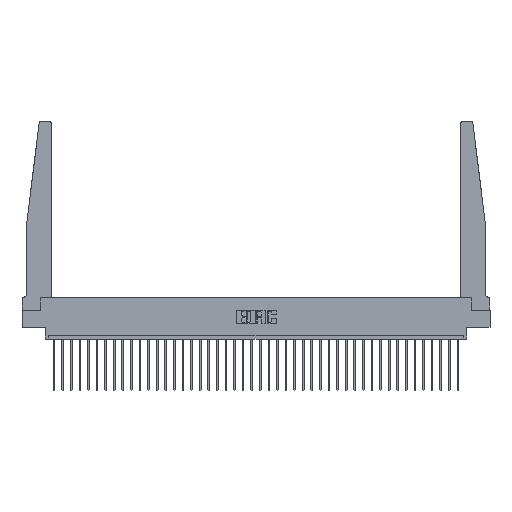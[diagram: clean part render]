
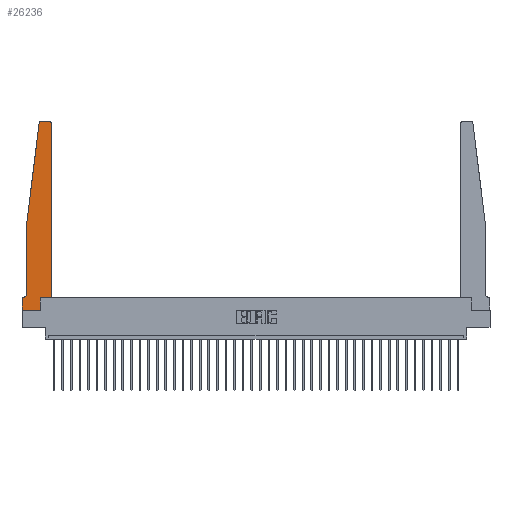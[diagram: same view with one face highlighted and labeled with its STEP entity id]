
A CAD part, top view. The second image highlights one B-rep face of the part: STEP entity #26236.
In plain terms, the highlighted planar face has unit normal (0, 0, 1).
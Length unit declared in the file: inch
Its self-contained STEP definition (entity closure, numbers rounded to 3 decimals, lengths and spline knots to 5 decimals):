
#259 = VECTOR ( 'NONE', #19504, 39.37008 ) ;
#717 = DIRECTION ( 'NONE',  ( 0., 0., 1. ) ) ;
#832 = ORIENTED_EDGE ( 'NONE', *, *, #10052, .T. ) ;
#1225 = VECTOR ( 'NONE', #22235, 39.37008 ) ;
#1252 = CARTESIAN_POINT ( 'NONE',  ( 0.015, 0.2375, 0.37 ) ) ;
#1656 = LINE ( 'NONE', #3688, #13061 ) ;
#1762 = EDGE_CURVE ( 'NONE', #8208, #15382, #31924, .T. ) ;
#2377 = CARTESIAN_POINT ( 'NONE',  ( 0., 0.1875, 0.37 ) ) ;
#2489 = LINE ( 'NONE', #8571, #6580 ) ;
#2525 = LINE ( 'NONE', #32675, #13989 ) ;
#3051 = ORIENTED_EDGE ( 'NONE', *, *, #27903, .T. ) ;
#3588 = ORIENTED_EDGE ( 'NONE', *, *, #18045, .T. ) ;
#3688 = CARTESIAN_POINT ( 'NONE',  ( 0., 0., 0.37 ) ) ;
#4366 = CARTESIAN_POINT ( 'NONE',  ( 0.425, 0.18, 0.37 ) ) ;
#4421 = CARTESIAN_POINT ( 'NONE',  ( 0.065, 0.1875, 0.37 ) ) ;
#4464 = VERTEX_POINT ( 'NONE', #14008 ) ;
#4659 = ORIENTED_EDGE ( 'NONE', *, *, #14331, .T. ) ;
#4847 = ORIENTED_EDGE ( 'NONE', *, *, #25561, .T. ) ;
#5660 = LINE ( 'NONE', #4421, #16729 ) ;
#5717 = VECTOR ( 'NONE', #11387, 39.37008 ) ;
#6159 = ORIENTED_EDGE ( 'NONE', *, *, #17369, .T. ) ;
#6405 = CARTESIAN_POINT ( 'NONE',  ( 0.065, 1.25, 0.37 ) ) ;
#6427 = VERTEX_POINT ( 'NONE', #22055 ) ;
#6580 = VECTOR ( 'NONE', #8460, 39.37008 ) ;
#7458 = DIRECTION ( 'NONE',  ( 0., 0., 1. ) ) ;
#7943 = VERTEX_POINT ( 'NONE', #2377 ) ;
#8208 = VERTEX_POINT ( 'NONE', #17450 ) ;
#8460 = DIRECTION ( 'NONE',  ( 0., -1., 0. ) ) ;
#8571 = CARTESIAN_POINT ( 'NONE',  ( 0.065, 1.25, 0.37 ) ) ;
#8684 = EDGE_CURVE ( 'NONE', #6427, #4464, #31117, .T. ) ;
#8844 = DIRECTION ( 'NONE',  ( 1., 0., 0. ) ) ;
#9470 = PLANE ( 'NONE',  #16461 ) ;
#9927 = CARTESIAN_POINT ( 'NONE',  ( 0.395, 2.75, 0.37 ) ) ;
#10019 = EDGE_CURVE ( 'NONE', #4464, #29358, #26160, .T. ) ;
#10052 = EDGE_CURVE ( 'NONE', #33023, #7943, #5660, .T. ) ;
#10509 = CARTESIAN_POINT ( 'NONE',  ( 0.24675, 2.72367, 0.37 ) ) ;
#11081 = AXIS2_PLACEMENT_3D ( 'NONE', #20601, #7458, #33244 ) ;
#11387 = DIRECTION ( 'NONE',  ( 0., 1., 0. ) ) ;
#11603 = CARTESIAN_POINT ( 'NONE',  ( 0.425, 0.18, 0.37 ) ) ;
#11612 = DIRECTION ( 'NONE',  ( -1., 0., 0. ) ) ;
#11889 = CIRCLE ( 'NONE', #26439, 0.03 ) ;
#13061 = VECTOR ( 'NONE', #8844, 39.37008 ) ;
#13989 = VECTOR ( 'NONE', #15220, 39.37008 ) ;
#14008 = CARTESIAN_POINT ( 'NONE',  ( 0.2605, 0.18, 0.37 ) ) ;
#14202 = CIRCLE ( 'NONE', #21307, 0.05 ) ;
#14331 = EDGE_CURVE ( 'NONE', #19979, #25881, #11889, .T. ) ;
#14965 = ORIENTED_EDGE ( 'NONE', *, *, #33420, .T. ) ;
#15220 = DIRECTION ( 'NONE',  ( 0., -1., 0. ) ) ;
#15255 = CARTESIAN_POINT ( 'NONE',  ( 0.27653, 2.75, 0.37 ) ) ;
#15382 = VERTEX_POINT ( 'NONE', #9927 ) ;
#15649 = CARTESIAN_POINT ( 'NONE',  ( 0.065, 1.25, 0.37 ) ) ;
#16461 = AXIS2_PLACEMENT_3D ( 'NONE', #27800, #30638, #30315 ) ;
#16729 = VECTOR ( 'NONE', #27637, 39.37008 ) ;
#16865 = CARTESIAN_POINT ( 'NONE',  ( 0.2605, 0.18, 0.37 ) ) ;
#17369 = EDGE_CURVE ( 'NONE', #25881, #17714, #22359, .T. ) ;
#17450 = CARTESIAN_POINT ( 'NONE',  ( 0.425, 2.72, 0.37 ) ) ;
#17714 = VERTEX_POINT ( 'NONE', #6405 ) ;
#18045 = EDGE_CURVE ( 'NONE', #15382, #19979, #30524, .T. ) ;
#18575 = DIRECTION ( 'NONE',  ( -0.122, -0.992, 0. ) ) ;
#19499 = VECTOR ( 'NONE', #18575, 39.37008 ) ;
#19504 = DIRECTION ( 'NONE',  ( -1., 0., 0. ) ) ;
#19979 = VERTEX_POINT ( 'NONE', #15255 ) ;
#20601 = CARTESIAN_POINT ( 'NONE',  ( 0.395, 2.72, 0.37 ) ) ;
#21089 = ORIENTED_EDGE ( 'NONE', *, *, #31214, .T. ) ;
#21303 = LINE ( 'NONE', #4366, #30741 ) ;
#21307 = AXIS2_PLACEMENT_3D ( 'NONE', #1252, #32337, #11612 ) ;
#22055 = CARTESIAN_POINT ( 'NONE',  ( 0.2605, 0., 0.37 ) ) ;
#22235 = DIRECTION ( 'NONE',  ( 1., 0., 0. ) ) ;
#22359 = LINE ( 'NONE', #15649, #19499 ) ;
#22473 = CARTESIAN_POINT ( 'NONE',  ( 0.25, 2.75, 0.37 ) ) ;
#22508 = DIRECTION ( 'NONE',  ( 0., 1., 0. ) ) ;
#22673 = VERTEX_POINT ( 'NONE', #24040 ) ;
#24040 = CARTESIAN_POINT ( 'NONE',  ( 0., 0., 0.37 ) ) ;
#24340 = CARTESIAN_POINT ( 'NONE',  ( 0.065, 0.2375, 0.37 ) ) ;
#25559 = ORIENTED_EDGE ( 'NONE', *, *, #10019, .T. ) ;
#25561 = EDGE_CURVE ( 'NONE', #22673, #6427, #1656, .T. ) ;
#25881 = VERTEX_POINT ( 'NONE', #10509 ) ;
#26160 = LINE ( 'NONE', #30391, #1225 ) ;
#26236 = ADVANCED_FACE ( 'NONE', ( #29433 ), #9470, .T. ) ;
#26439 = AXIS2_PLACEMENT_3D ( 'NONE', #32019, #717, #31905 ) ;
#27637 = DIRECTION ( 'NONE',  ( -1., 0., 0. ) ) ;
#27800 = CARTESIAN_POINT ( 'NONE',  ( 0., 0.1875, 0.37 ) ) ;
#27903 = EDGE_CURVE ( 'NONE', #32068, #33023, #14202, .T. ) ;
#28403 = ORIENTED_EDGE ( 'NONE', *, *, #8684, .T. ) ;
#28504 = EDGE_LOOP ( 'NONE', ( #3588, #4659, #6159, #30066, #3051, #832, #21089, #4847, #28403, #25559, #14965, #29049 ) ) ;
#29049 = ORIENTED_EDGE ( 'NONE', *, *, #1762, .T. ) ;
#29358 = VERTEX_POINT ( 'NONE', #11603 ) ;
#29433 = FACE_OUTER_BOUND ( 'NONE', #28504, .T. ) ;
#30066 = ORIENTED_EDGE ( 'NONE', *, *, #31441, .T. ) ;
#30315 = DIRECTION ( 'NONE',  ( 1., 0., 0. ) ) ;
#30391 = CARTESIAN_POINT ( 'NONE',  ( 0.425, 0.18, 0.37 ) ) ;
#30524 = LINE ( 'NONE', #22473, #259 ) ;
#30638 = DIRECTION ( 'NONE',  ( 0., 0., 1. ) ) ;
#30741 = VECTOR ( 'NONE', #22508, 39.37008 ) ;
#31117 = LINE ( 'NONE', #16865, #5717 ) ;
#31214 = EDGE_CURVE ( 'NONE', #7943, #22673, #2525, .T. ) ;
#31441 = EDGE_CURVE ( 'NONE', #17714, #32068, #2489, .T. ) ;
#31691 = CARTESIAN_POINT ( 'NONE',  ( 0.015, 0.1875, 0.37 ) ) ;
#31905 = DIRECTION ( 'NONE',  ( 1., 0., 0. ) ) ;
#31924 = CIRCLE ( 'NONE', #11081, 0.03 ) ;
#32019 = CARTESIAN_POINT ( 'NONE',  ( 0.27653, 2.72, 0.37 ) ) ;
#32068 = VERTEX_POINT ( 'NONE', #24340 ) ;
#32337 = DIRECTION ( 'NONE',  ( 0., 0., -1. ) ) ;
#32675 = CARTESIAN_POINT ( 'NONE',  ( 0., 0., 0.37 ) ) ;
#33023 = VERTEX_POINT ( 'NONE', #31691 ) ;
#33244 = DIRECTION ( 'NONE',  ( 1., 0., 0. ) ) ;
#33420 = EDGE_CURVE ( 'NONE', #29358, #8208, #21303, .T. ) ;
